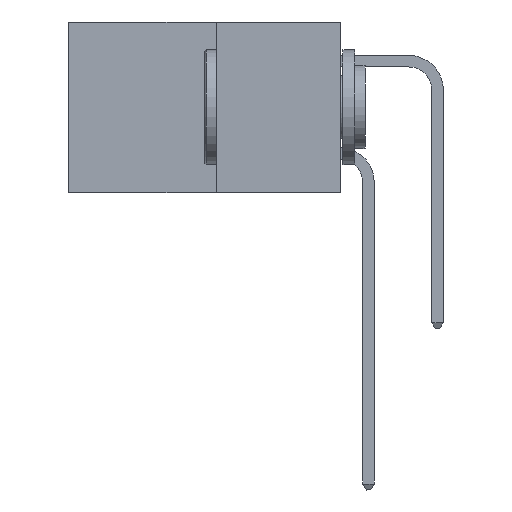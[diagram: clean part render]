
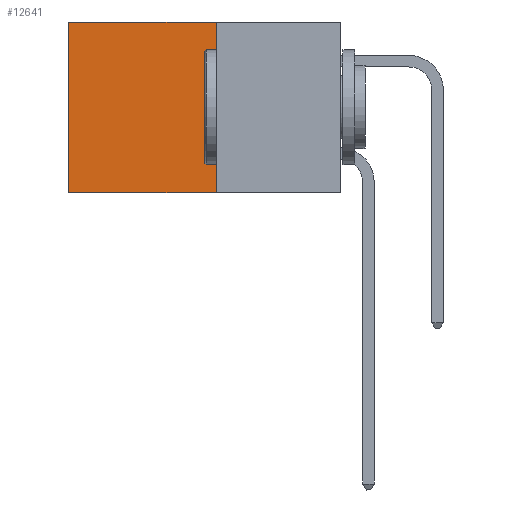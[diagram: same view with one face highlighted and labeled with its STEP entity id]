
A CAD part, left-side view. The second image highlights one B-rep face of the part: STEP entity #12641.
In plain terms, the highlighted planar face has unit normal (-1, 0, 0).
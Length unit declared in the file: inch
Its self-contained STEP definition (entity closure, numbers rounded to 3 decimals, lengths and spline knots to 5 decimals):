
#1198 = VECTOR ( 'NONE', #12267, 39.37008 ) ;
#1288 = CARTESIAN_POINT ( 'NONE',  ( 0.277, 0.27, -0.37 ) ) ;
#2325 = PLANE ( 'NONE',  #12512 ) ;
#2378 = CARTESIAN_POINT ( 'NONE',  ( 0.277, 0.27, 0. ) ) ;
#2686 = CARTESIAN_POINT ( 'NONE',  ( 0.277, 0.59, -0.37 ) ) ;
#3748 = ORIENTED_EDGE ( 'NONE', *, *, #10718, .T. ) ;
#4403 = FACE_OUTER_BOUND ( 'NONE', #20043, .T. ) ;
#4865 = VECTOR ( 'NONE', #21545, 39.37008 ) ;
#6313 = LINE ( 'NONE', #2686, #1198 ) ;
#6726 = CARTESIAN_POINT ( 'NONE',  ( 0.277, 0.59, -0.37 ) ) ;
#7007 = VERTEX_POINT ( 'NONE', #6726 ) ;
#7069 = VERTEX_POINT ( 'NONE', #8640 ) ;
#7646 = EDGE_CURVE ( 'NONE', #10316, #7069, #20779, .T. ) ;
#7748 = ORIENTED_EDGE ( 'NONE', *, *, #24127, .T. ) ;
#8131 = CARTESIAN_POINT ( 'NONE',  ( 0.277, 0.27, -0.37 ) ) ;
#8640 = CARTESIAN_POINT ( 'NONE',  ( 0.277, 0.27, -0.37 ) ) ;
#9044 = VERTEX_POINT ( 'NONE', #13512 ) ;
#9958 = LINE ( 'NONE', #2378, #4865 ) ;
#10041 = DIRECTION ( 'NONE',  ( 0., 0., -1. ) ) ;
#10177 = EDGE_CURVE ( 'NONE', #7069, #7007, #13849, .T. ) ;
#10316 = VERTEX_POINT ( 'NONE', #20767 ) ;
#10633 = VECTOR ( 'NONE', #23957, 39.37008 ) ;
#10718 = EDGE_CURVE ( 'NONE', #9044, #7007, #6313, .T. ) ;
#10771 = DIRECTION ( 'NONE',  ( 0., 1., 0. ) ) ;
#12267 = DIRECTION ( 'NONE',  ( 0., 0., -1. ) ) ;
#12512 = AXIS2_PLACEMENT_3D ( 'NONE', #8131, #21499, #10041 ) ;
#12641 = ADVANCED_FACE ( 'NONE', ( #4403 ), #2325, .F. ) ;
#13512 = CARTESIAN_POINT ( 'NONE',  ( 0.277, 0.59, 0. ) ) ;
#13849 = LINE ( 'NONE', #14736, #18887 ) ;
#14736 = CARTESIAN_POINT ( 'NONE',  ( 0.277, 0.27, -0.37 ) ) ;
#18887 = VECTOR ( 'NONE', #10771, 39.37008 ) ;
#20043 = EDGE_LOOP ( 'NONE', ( #3748, #22297, #21601, #7748 ) ) ;
#20767 = CARTESIAN_POINT ( 'NONE',  ( 0.277, 0.27, 0. ) ) ;
#20779 = LINE ( 'NONE', #1288, #10633 ) ;
#21499 = DIRECTION ( 'NONE',  ( 1., 0., 0. ) ) ;
#21545 = DIRECTION ( 'NONE',  ( 0., 1., 0. ) ) ;
#21601 = ORIENTED_EDGE ( 'NONE', *, *, #7646, .F. ) ;
#22297 = ORIENTED_EDGE ( 'NONE', *, *, #10177, .F. ) ;
#23957 = DIRECTION ( 'NONE',  ( 0., 0., -1. ) ) ;
#24127 = EDGE_CURVE ( 'NONE', #10316, #9044, #9958, .T. ) ;
